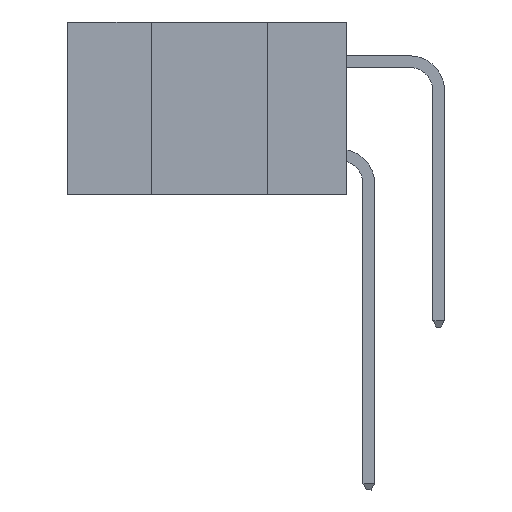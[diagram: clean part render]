
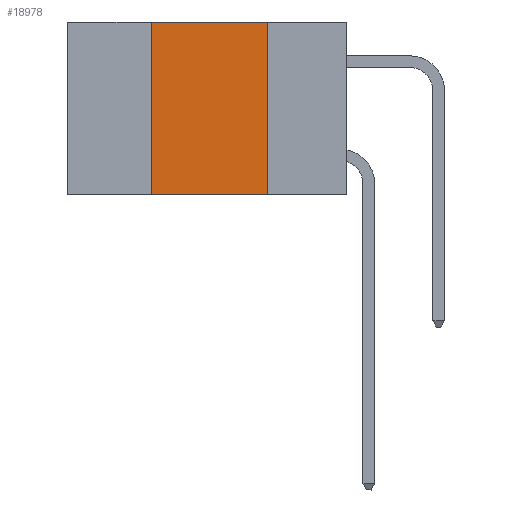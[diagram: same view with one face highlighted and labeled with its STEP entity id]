
A CAD part, left-side view. The second image highlights one B-rep face of the part: STEP entity #18978.
In plain terms, the highlighted planar face has unit normal (-1, 0, 0).
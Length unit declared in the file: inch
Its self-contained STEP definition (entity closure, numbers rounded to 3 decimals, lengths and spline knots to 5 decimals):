
#1497 = CARTESIAN_POINT ( 'NONE',  ( 0., 0.17, 0. ) ) ;
#3020 = EDGE_CURVE ( 'NONE', #42073, #34012, #18388, .T. ) ;
#4937 = LINE ( 'NONE', #1497, #5422 ) ;
#5422 = VECTOR ( 'NONE', #34083, 39.37008 ) ;
#5632 = LINE ( 'NONE', #5847, #32551 ) ;
#5847 = CARTESIAN_POINT ( 'NONE',  ( 0., 0.6, -0.37 ) ) ;
#9437 = ORIENTED_EDGE ( 'NONE', *, *, #29259, .T. ) ;
#11912 = PLANE ( 'NONE',  #26563 ) ;
#12197 = ORIENTED_EDGE ( 'NONE', *, *, #26061, .F. ) ;
#17442 = DIRECTION ( 'NONE',  ( 0., 0., 1. ) ) ;
#18388 = LINE ( 'NONE', #37700, #20944 ) ;
#18894 = DIRECTION ( 'NONE',  ( 0., -1., 0. ) ) ;
#18978 = ADVANCED_FACE ( 'NONE', ( #28654 ), #11912, .F. ) ;
#19197 = ORIENTED_EDGE ( 'NONE', *, *, #34958, .F. ) ;
#19990 = CARTESIAN_POINT ( 'NONE',  ( 0., 0.42, -0.37 ) ) ;
#20944 = VECTOR ( 'NONE', #30467, 39.37008 ) ;
#21297 = LINE ( 'NONE', #24522, #40575 ) ;
#21779 = DIRECTION ( 'NONE',  ( 1., 0., 0. ) ) ;
#22651 = CARTESIAN_POINT ( 'NONE',  ( 0., 0.42, 0. ) ) ;
#24522 = CARTESIAN_POINT ( 'NONE',  ( 0., 0.42, 0. ) ) ;
#24749 = CARTESIAN_POINT ( 'NONE',  ( 0., 0.17, 0. ) ) ;
#25001 = CARTESIAN_POINT ( 'NONE',  ( 0., 0.6, 0. ) ) ;
#26061 = EDGE_CURVE ( 'NONE', #39715, #42073, #21297, .T. ) ;
#26165 = VERTEX_POINT ( 'NONE', #28586 ) ;
#26563 = AXIS2_PLACEMENT_3D ( 'NONE', #25001, #21779, #28230 ) ;
#28230 = DIRECTION ( 'NONE',  ( 0., 0., -1. ) ) ;
#28586 = CARTESIAN_POINT ( 'NONE',  ( 0., 0.17, -0.37 ) ) ;
#28654 = FACE_OUTER_BOUND ( 'NONE', #34712, .T. ) ;
#29259 = EDGE_CURVE ( 'NONE', #39715, #26165, #5632, .T. ) ;
#30467 = DIRECTION ( 'NONE',  ( 0., -1., 0. ) ) ;
#32551 = VECTOR ( 'NONE', #18894, 39.37008 ) ;
#34012 = VERTEX_POINT ( 'NONE', #24749 ) ;
#34083 = DIRECTION ( 'NONE',  ( 0., 0., -1. ) ) ;
#34712 = EDGE_LOOP ( 'NONE', ( #19197, #35970, #12197, #9437 ) ) ;
#34958 = EDGE_CURVE ( 'NONE', #34012, #26165, #4937, .T. ) ;
#35970 = ORIENTED_EDGE ( 'NONE', *, *, #3020, .F. ) ;
#37700 = CARTESIAN_POINT ( 'NONE',  ( 0., 0.6, 0. ) ) ;
#39715 = VERTEX_POINT ( 'NONE', #19990 ) ;
#40575 = VECTOR ( 'NONE', #17442, 39.37008 ) ;
#42073 = VERTEX_POINT ( 'NONE', #22651 ) ;
